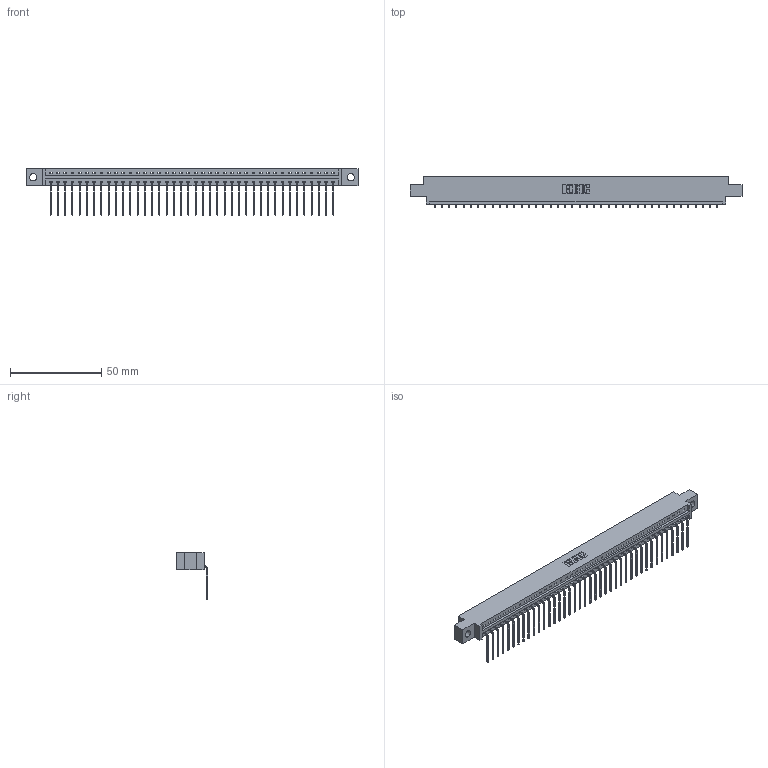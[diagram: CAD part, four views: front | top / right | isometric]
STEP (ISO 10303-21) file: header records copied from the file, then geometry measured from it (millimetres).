
FILE_DESCRIPTION (( 'STEP AP203' ), '1' );
FILE_NAME ('337-040-559-604.STEP', '2019-10-01T20:10:39', ( '' ), ( '' ), 'SwSTEP 2.0', 'SolidWorks 2016', '' );
FILE_SCHEMA (( 'CONFIG_CONTROL_DESIGN' ));
Length unit declared in the file: inch
Products named in the file (3): 337-040-559-604; 337 Part_0.170 Offset - 0.156 Dia-TH; 345-292-001_558 559 Tail - 1
Assembly tree (41 placements, depth 2):
  337-040-559-604
    337 Part_0.170 Offset - 0.156 Dia-TH
    345-292-001_558 559 Tail - 1  x40
Bounding box: 181.51 x 17.09 x 25.53 mm (x, y, z)
Volume: 18767.6 mm3; surface area: 20092.9 mm2
Topology: 41 solids, 41 shells, 2678 faces, 8083 edges, 5334 vertices
Faces by surface type: plane 1994, cylinder 684
Entity records: 30211 total; most frequent: CARTESIAN_POINT 5270, ORIENTED_EDGE 5246, DIRECTION 4439, EDGE_CURVE 2623, VECTOR 2495, LINE 2495, VERTEX_POINT 1746, AXIS2_PLACEMENT_3D 972
